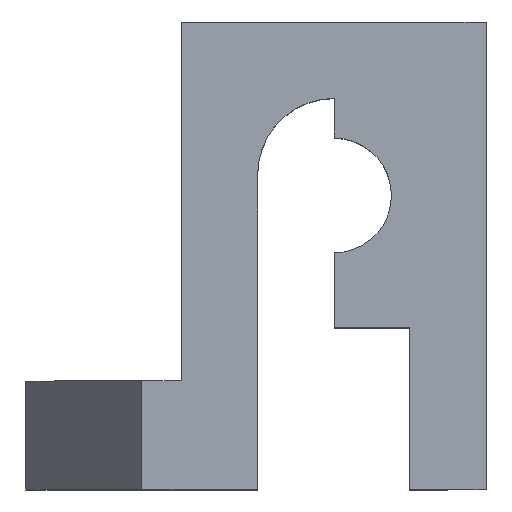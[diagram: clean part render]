
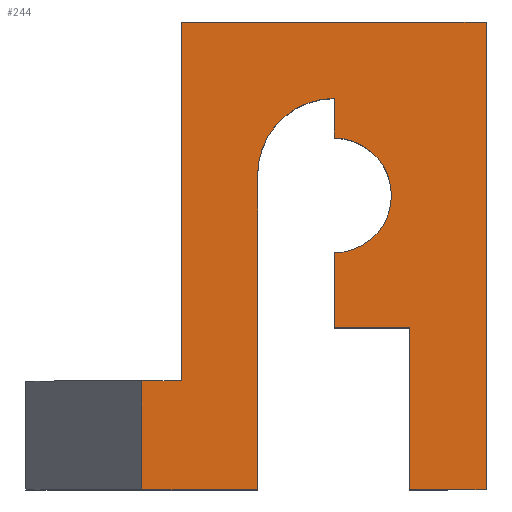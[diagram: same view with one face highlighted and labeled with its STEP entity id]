
A CAD part, top view. The second image highlights one B-rep face of the part: STEP entity #244.
In plain terms, the highlighted planar face has unit normal (0, 0, 1).
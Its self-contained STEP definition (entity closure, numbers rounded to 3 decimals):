
#75=CARTESIAN_POINT('',(-10.03,2.85,4.0));
#76=VERTEX_POINT('',#75);
#91=CARTESIAN_POINT('',(-10.03,0.0,4.0));
#92=VERTEX_POINT('',#91);
#99=CARTESIAN_POINT('',(-10.03,2.85,4.0));
#100=DIRECTION('',(0.0,-1.0,0.0));
#101=VECTOR('',#100,2.85);
#102=LINE('',#99,#101);
#103=EDGE_CURVE('',#76,#92,#102,.T.);
#114=CARTESIAN_POINT('',(-9.0,2.85,4.0));
#115=VERTEX_POINT('',#114);
#116=CARTESIAN_POINT('',(-9.0,2.85,4.0));
#117=DIRECTION('',(-1.0,0.0,0.0));
#118=VECTOR('',#117,1.03);
#119=LINE('',#116,#118);
#120=EDGE_CURVE('',#115,#76,#119,.T.);
#139=CARTESIAN_POINT('',(-5.983,5.597,4.0));
#140=DIRECTION('',(0.0,0.0,1.0));
#141=DIRECTION('',(1.0,0.0,0.0));
#142=AXIS2_PLACEMENT_3D('',#139,#140,#141);
#143=PLANE('',#142);
#144=ORIENTED_EDGE('',*,*,#103,.T.);
#145=CARTESIAN_POINT('',(-7.0,0.0,4.0));
#146=VERTEX_POINT('',#145);
#147=CARTESIAN_POINT('',(-10.03,0.0,4.0));
#148=DIRECTION('',(1.0,0.0,0.0));
#149=VECTOR('',#148,3.03);
#150=LINE('',#147,#149);
#151=EDGE_CURVE('',#92,#146,#150,.T.);
#152=ORIENTED_EDGE('',*,*,#151,.T.);
#153=CARTESIAN_POINT('',(-7.0,8.235,4.0));
#154=VERTEX_POINT('',#153);
#155=CARTESIAN_POINT('',(-7.0,0.0,4.0));
#156=DIRECTION('',(0.0,1.0,0.0));
#157=VECTOR('',#156,8.235);
#158=LINE('',#155,#157);
#159=EDGE_CURVE('',#146,#154,#158,.T.);
#160=ORIENTED_EDGE('',*,*,#159,.T.);
#161=CARTESIAN_POINT('',(-5.,10.235,4.0));
#162=VERTEX_POINT('',#161);
#163=CARTESIAN_POINT('',(-5.,8.235,4.0));
#164=DIRECTION('',(0.0,0.0,-1.0));
#165=DIRECTION('',(0.0,-1.0,0.0));
#166=AXIS2_PLACEMENT_3D('',#163,#164,#165);
#167=CIRCLE('',#166,2.0);
#168=EDGE_CURVE('',#154,#162,#167,.T.);
#169=ORIENTED_EDGE('',*,*,#168,.T.);
#170=CARTESIAN_POINT('',(-5.0,9.198,4.0));
#171=VERTEX_POINT('',#170);
#172=CARTESIAN_POINT('',(-5.0,10.235,4.0));
#173=DIRECTION('',(0.0,-1.0,0.0));
#174=VECTOR('',#173,1.037);
#175=LINE('',#172,#174);
#176=EDGE_CURVE('',#162,#171,#175,.T.);
#177=ORIENTED_EDGE('',*,*,#176,.T.);
#178=CARTESIAN_POINT('',(-5.0,6.198,4.0));
#179=VERTEX_POINT('',#178);
#180=CARTESIAN_POINT('',(-5.0,7.698,4.0));
#181=DIRECTION('',(0.0,0.0,-1.0));
#182=DIRECTION('',(0.0,1.0,0.0));
#183=AXIS2_PLACEMENT_3D('',#180,#181,#182);
#184=CIRCLE('',#183,1.5);
#185=EDGE_CURVE('',#171,#179,#184,.T.);
#186=ORIENTED_EDGE('',*,*,#185,.T.);
#187=CARTESIAN_POINT('',(-5.,4.235,4.0));
#188=VERTEX_POINT('',#187);
#189=CARTESIAN_POINT('',(-5.0,6.198,4.0));
#190=DIRECTION('',(0.0,-1.0,0.0));
#191=VECTOR('',#190,1.963);
#192=LINE('',#189,#191);
#193=EDGE_CURVE('',#179,#188,#192,.T.);
#194=ORIENTED_EDGE('',*,*,#193,.T.);
#195=CARTESIAN_POINT('',(-3.024,4.235,4.0));
#196=VERTEX_POINT('',#195);
#197=CARTESIAN_POINT('',(-5.,4.235,4.0));
#198=DIRECTION('',(1.0,0.0,0.0));
#199=VECTOR('',#198,1.976);
#200=LINE('',#197,#199);
#201=EDGE_CURVE('',#188,#196,#200,.T.);
#202=ORIENTED_EDGE('',*,*,#201,.T.);
#203=CARTESIAN_POINT('',(-3.024,0.0,4.0));
#204=VERTEX_POINT('',#203);
#205=CARTESIAN_POINT('',(-3.024,4.235,4.0));
#206=DIRECTION('',(0.0,-1.0,0.0));
#207=VECTOR('',#206,4.235);
#208=LINE('',#205,#207);
#209=EDGE_CURVE('',#196,#204,#208,.T.);
#210=ORIENTED_EDGE('',*,*,#209,.T.);
#211=CARTESIAN_POINT('',(-1.024,0.,4.0));
#212=VERTEX_POINT('',#211);
#213=CARTESIAN_POINT('',(-3.024,0.,4.0));
#214=DIRECTION('',(1.0,0.0,0.0));
#215=VECTOR('',#214,2.);
#216=LINE('',#213,#215);
#217=EDGE_CURVE('',#204,#212,#216,.T.);
#218=ORIENTED_EDGE('',*,*,#217,.T.);
#219=CARTESIAN_POINT('',(-1.024,12.235,4.0));
#220=VERTEX_POINT('',#219);
#221=CARTESIAN_POINT('',(-1.024,0.,4.0));
#222=DIRECTION('',(0.0,1.0,0.0));
#223=VECTOR('',#222,12.235);
#224=LINE('',#221,#223);
#225=EDGE_CURVE('',#212,#220,#224,.T.);
#226=ORIENTED_EDGE('',*,*,#225,.T.);
#227=CARTESIAN_POINT('',(-9.0,12.235,4.0));
#228=VERTEX_POINT('',#227);
#229=CARTESIAN_POINT('',(-1.024,12.235,4.0));
#230=DIRECTION('',(-1.0,0.0,0.0));
#231=VECTOR('',#230,7.976);
#232=LINE('',#229,#231);
#233=EDGE_CURVE('',#220,#228,#232,.T.);
#234=ORIENTED_EDGE('',*,*,#233,.T.);
#235=CARTESIAN_POINT('',(-9.0,12.235,4.0));
#236=DIRECTION('',(0.0,-1.0,0.0));
#237=VECTOR('',#236,9.386);
#238=LINE('',#235,#237);
#239=EDGE_CURVE('',#228,#115,#238,.T.);
#240=ORIENTED_EDGE('',*,*,#239,.T.);
#241=ORIENTED_EDGE('',*,*,#120,.T.);
#242=EDGE_LOOP('',(#144,#152,#160,#169,#177,#186,#194,#202,#210,#218,#226,#234,#240,#241));
#243=FACE_OUTER_BOUND('',#242,.T.);
#244=ADVANCED_FACE('',(#243),#143,.T.);
